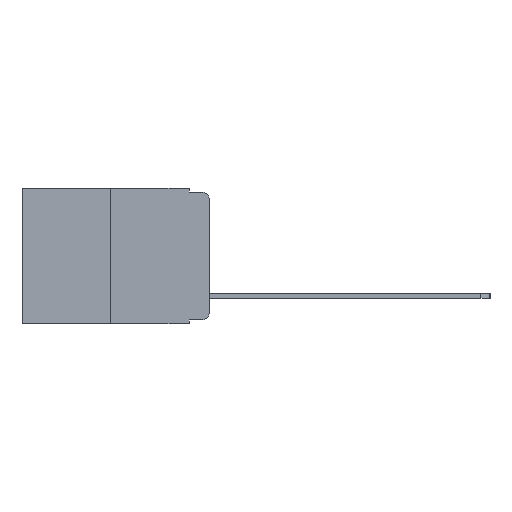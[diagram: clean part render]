
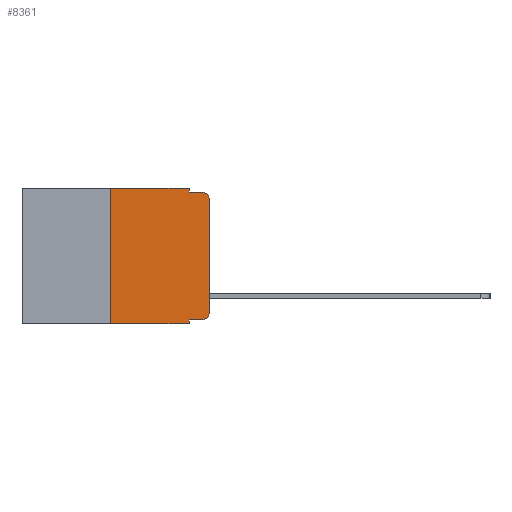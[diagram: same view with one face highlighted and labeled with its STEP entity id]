
A CAD part, left-side view. The second image highlights one B-rep face of the part: STEP entity #8361.
In plain terms, the highlighted planar face has unit normal (-1, 0, 0).
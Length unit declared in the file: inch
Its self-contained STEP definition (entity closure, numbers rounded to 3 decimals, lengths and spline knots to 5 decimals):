
#2 = CARTESIAN_POINT ( 'NONE',  ( 0., 0.051, 0. ) ) ;
#98 = CARTESIAN_POINT ( 'NONE',  ( 0., 0.051, 0. ) ) ;
#272 = VERTEX_POINT ( 'NONE', #18547 ) ;
#276 = VERTEX_POINT ( 'NONE', #3864 ) ;
#455 = ORIENTED_EDGE ( 'NONE', *, *, #2193, .T. ) ;
#554 = VECTOR ( 'NONE', #12555, 39.37008 ) ;
#588 = VERTEX_POINT ( 'NONE', #12363 ) ;
#842 = CARTESIAN_POINT ( 'NONE',  ( 0., 0.051, -0.333 ) ) ;
#1676 = DIRECTION ( 'NONE',  ( 0., 0., -1. ) ) ;
#1700 = VERTEX_POINT ( 'NONE', #12835 ) ;
#1709 = CARTESIAN_POINT ( 'NONE',  ( 0., 0.051, -0.01 ) ) ;
#1818 = ORIENTED_EDGE ( 'NONE', *, *, #9424, .F. ) ;
#2193 = EDGE_CURVE ( 'NONE', #10610, #272, #19121, .T. ) ;
#2235 = ORIENTED_EDGE ( 'NONE', *, *, #6796, .T. ) ;
#2318 = ORIENTED_EDGE ( 'NONE', *, *, #4249, .T. ) ;
#2360 = AXIS2_PLACEMENT_3D ( 'NONE', #15200, #5515, #16699 ) ;
#2887 = VECTOR ( 'NONE', #15292, 39.37008 ) ;
#3107 = ORIENTED_EDGE ( 'NONE', *, *, #17390, .F. ) ;
#3118 = DIRECTION ( 'NONE',  ( 1., 0., 0. ) ) ;
#3350 = ORIENTED_EDGE ( 'NONE', *, *, #7505, .F. ) ;
#3771 = DIRECTION ( 'NONE',  ( 0., 0., 1. ) ) ;
#3864 = CARTESIAN_POINT ( 'NONE',  ( 0., 0., -0.03 ) ) ;
#3910 = DIRECTION ( 'NONE',  ( 0., 0., 1. ) ) ;
#4249 = EDGE_CURVE ( 'NONE', #588, #276, #5819, .T. ) ;
#4693 = CARTESIAN_POINT ( 'NONE',  ( 0., 0.25, 0. ) ) ;
#5200 = DIRECTION ( 'NONE',  ( 0., 0., -1. ) ) ;
#5281 = VECTOR ( 'NONE', #3771, 39.37008 ) ;
#5515 = DIRECTION ( 'NONE',  ( -1., 0., 0. ) ) ;
#5653 = LINE ( 'NONE', #98, #17848 ) ;
#5819 = LINE ( 'NONE', #18242, #5281 ) ;
#6556 = LINE ( 'NONE', #2, #11990 ) ;
#6796 = EDGE_CURVE ( 'NONE', #276, #1700, #15751, .T. ) ;
#7098 = LINE ( 'NONE', #15270, #14641 ) ;
#7135 = ORIENTED_EDGE ( 'NONE', *, *, #8538, .T. ) ;
#7326 = DIRECTION ( 'NONE',  ( 0., -1., 0. ) ) ;
#7359 = CARTESIAN_POINT ( 'NONE',  ( 0., 0.02, -0.03 ) ) ;
#7450 = LINE ( 'NONE', #15231, #2887 ) ;
#7505 = EDGE_CURVE ( 'NONE', #16306, #16858, #5653, .T. ) ;
#8361 = ADVANCED_FACE ( 'NONE', ( #11643 ), #11539, .F. ) ;
#8368 = CARTESIAN_POINT ( 'NONE',  ( 0., 0.25, -0.343 ) ) ;
#8453 = ORIENTED_EDGE ( 'NONE', *, *, #10310, .T. ) ;
#8496 = VECTOR ( 'NONE', #3910, 39.37008 ) ;
#8538 = EDGE_CURVE ( 'NONE', #13729, #588, #14503, .T. ) ;
#8540 = AXIS2_PLACEMENT_3D ( 'NONE', #20613, #3118, #14615 ) ;
#8749 = ORIENTED_EDGE ( 'NONE', *, *, #15565, .F. ) ;
#9065 = DIRECTION ( 'NONE',  ( 0., 0., -1. ) ) ;
#9368 = ORIENTED_EDGE ( 'NONE', *, *, #18725, .F. ) ;
#9424 = EDGE_CURVE ( 'NONE', #10610, #16668, #20346, .T. ) ;
#10011 = CARTESIAN_POINT ( 'NONE',  ( 0., 0.02, -0.333 ) ) ;
#10310 = EDGE_CURVE ( 'NONE', #13884, #13729, #17330, .T. ) ;
#10610 = VERTEX_POINT ( 'NONE', #8368 ) ;
#11539 = PLANE ( 'NONE',  #8540 ) ;
#11643 = FACE_OUTER_BOUND ( 'NONE', #15247, .T. ) ;
#11990 = VECTOR ( 'NONE', #1676, 39.37008 ) ;
#12363 = CARTESIAN_POINT ( 'NONE',  ( 0., 0., -0.313 ) ) ;
#12555 = DIRECTION ( 'NONE',  ( 0., -1., 0. ) ) ;
#12835 = CARTESIAN_POINT ( 'NONE',  ( 0., 0.02, -0.01 ) ) ;
#13348 = CARTESIAN_POINT ( 'NONE',  ( 0., 0.473, -0.343 ) ) ;
#13370 = DIRECTION ( 'NONE',  ( 0., -1., 0. ) ) ;
#13729 = VERTEX_POINT ( 'NONE', #10011 ) ;
#13814 = CARTESIAN_POINT ( 'NONE',  ( 0., 0.25, 0. ) ) ;
#13884 = VERTEX_POINT ( 'NONE', #14959 ) ;
#14503 = CIRCLE ( 'NONE', #2360, 0.02 ) ;
#14615 = DIRECTION ( 'NONE',  ( 0., 0., -1. ) ) ;
#14641 = VECTOR ( 'NONE', #7326, 39.37008 ) ;
#14959 = CARTESIAN_POINT ( 'NONE',  ( 0., 0.051, -0.333 ) ) ;
#15200 = CARTESIAN_POINT ( 'NONE',  ( 0., 0.02, -0.313 ) ) ;
#15231 = CARTESIAN_POINT ( 'NONE',  ( 0., 0.473, 0. ) ) ;
#15247 = EDGE_LOOP ( 'NONE', ( #2318, #2235, #3107, #3350, #8749, #1818, #455, #9368, #8453, #7135 ) ) ;
#15270 = CARTESIAN_POINT ( 'NONE',  ( 0., 0.051, -0.01 ) ) ;
#15292 = DIRECTION ( 'NONE',  ( 0., -1., 0. ) ) ;
#15565 = EDGE_CURVE ( 'NONE', #16668, #16306, #7450, .T. ) ;
#15751 = CIRCLE ( 'NONE', #19330, 0.02 ) ;
#16306 = VERTEX_POINT ( 'NONE', #19808 ) ;
#16668 = VERTEX_POINT ( 'NONE', #4693 ) ;
#16699 = DIRECTION ( 'NONE',  ( 0., 0., -1. ) ) ;
#16858 = VERTEX_POINT ( 'NONE', #1709 ) ;
#17330 = LINE ( 'NONE', #842, #554 ) ;
#17390 = EDGE_CURVE ( 'NONE', #16858, #1700, #7098, .T. ) ;
#17848 = VECTOR ( 'NONE', #5200, 39.37008 ) ;
#18242 = CARTESIAN_POINT ( 'NONE',  ( 0., 0., 0. ) ) ;
#18332 = DIRECTION ( 'NONE',  ( -1., 0., 0. ) ) ;
#18547 = CARTESIAN_POINT ( 'NONE',  ( 0., 0.051, -0.343 ) ) ;
#18725 = EDGE_CURVE ( 'NONE', #13884, #272, #6556, .T. ) ;
#19121 = LINE ( 'NONE', #13348, #19578 ) ;
#19330 = AXIS2_PLACEMENT_3D ( 'NONE', #7359, #18332, #9065 ) ;
#19578 = VECTOR ( 'NONE', #13370, 39.37008 ) ;
#19808 = CARTESIAN_POINT ( 'NONE',  ( 0., 0.051, 0. ) ) ;
#20346 = LINE ( 'NONE', #13814, #8496 ) ;
#20613 = CARTESIAN_POINT ( 'NONE',  ( 0., 0.473, 0. ) ) ;
